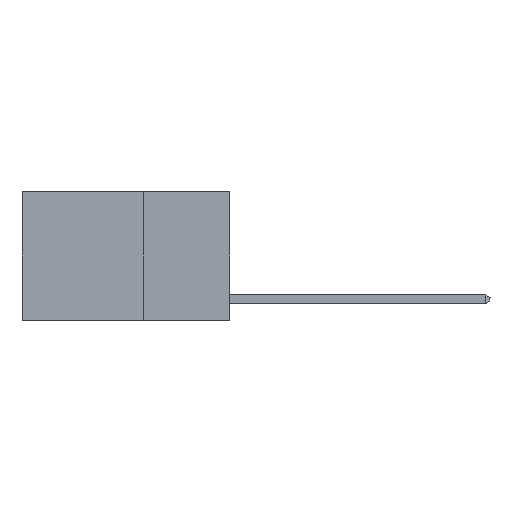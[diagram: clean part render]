
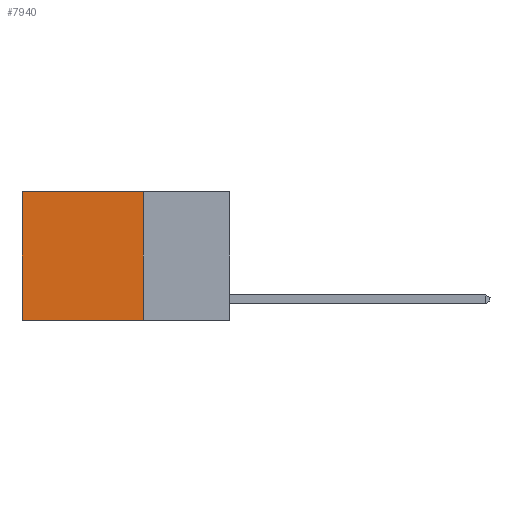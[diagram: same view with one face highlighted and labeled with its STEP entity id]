
A CAD part, left-side view. The second image highlights one B-rep face of the part: STEP entity #7940.
In plain terms, the highlighted planar face has unit normal (-1, 0, 0).
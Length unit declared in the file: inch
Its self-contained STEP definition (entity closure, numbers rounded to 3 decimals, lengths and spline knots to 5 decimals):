
#1257 = VECTOR ( 'NONE', #20396, 39.37008 ) ;
#1799 = CARTESIAN_POINT ( 'NONE',  ( 0.2625, 0.6, 0. ) ) ;
#1955 = VECTOR ( 'NONE', #23420, 39.37008 ) ;
#2367 = ORIENTED_EDGE ( 'NONE', *, *, #23529, .T. ) ;
#2864 = VECTOR ( 'NONE', #13400, 39.37008 ) ;
#3871 = VERTEX_POINT ( 'NONE', #1799 ) ;
#3995 = DIRECTION ( 'NONE',  ( 0., 0., -1. ) ) ;
#4753 = CARTESIAN_POINT ( 'NONE',  ( 0.2625, 0.25, 0. ) ) ;
#6244 = CARTESIAN_POINT ( 'NONE',  ( 0.2625, 0.25, 0. ) ) ;
#7244 = CARTESIAN_POINT ( 'NONE',  ( 0.2625, 0.6, -0.37 ) ) ;
#7940 = ADVANCED_FACE ( 'NONE', ( #25954 ), #25672, .F. ) ;
#8669 = LINE ( 'NONE', #17328, #1955 ) ;
#9231 = VERTEX_POINT ( 'NONE', #17182 ) ;
#9252 = EDGE_CURVE ( 'NONE', #9231, #19351, #8669, .T. ) ;
#9259 = VERTEX_POINT ( 'NONE', #19178 ) ;
#9519 = LINE ( 'NONE', #22286, #19576 ) ;
#10224 = DIRECTION ( 'NONE',  ( 1., 0., 0. ) ) ;
#13400 = DIRECTION ( 'NONE',  ( 0., 0., -1. ) ) ;
#14044 = LINE ( 'NONE', #26610, #1257 ) ;
#14243 = EDGE_CURVE ( 'NONE', #3871, #19351, #14044, .T. ) ;
#15891 = ORIENTED_EDGE ( 'NONE', *, *, #24357, .F. ) ;
#15917 = DIRECTION ( 'NONE',  ( 0., 1., 0. ) ) ;
#16016 = EDGE_LOOP ( 'NONE', ( #24887, #25338, #15891, #2367 ) ) ;
#17182 = CARTESIAN_POINT ( 'NONE',  ( 0.2625, 0.25, -0.37 ) ) ;
#17328 = CARTESIAN_POINT ( 'NONE',  ( 0.2625, 0.25, -0.37 ) ) ;
#19178 = CARTESIAN_POINT ( 'NONE',  ( 0.2625, 0.25, 0. ) ) ;
#19351 = VERTEX_POINT ( 'NONE', #7244 ) ;
#19576 = VECTOR ( 'NONE', #15917, 39.37008 ) ;
#19834 = AXIS2_PLACEMENT_3D ( 'NONE', #6244, #10224, #3995 ) ;
#20396 = DIRECTION ( 'NONE',  ( 0., 0., -1. ) ) ;
#22286 = CARTESIAN_POINT ( 'NONE',  ( 0.2625, 0.25, 0. ) ) ;
#23420 = DIRECTION ( 'NONE',  ( 0., 1., 0. ) ) ;
#23529 = EDGE_CURVE ( 'NONE', #9259, #3871, #9519, .T. ) ;
#24177 = LINE ( 'NONE', #4753, #2864 ) ;
#24357 = EDGE_CURVE ( 'NONE', #9259, #9231, #24177, .T. ) ;
#24887 = ORIENTED_EDGE ( 'NONE', *, *, #14243, .T. ) ;
#25338 = ORIENTED_EDGE ( 'NONE', *, *, #9252, .F. ) ;
#25672 = PLANE ( 'NONE',  #19834 ) ;
#25954 = FACE_OUTER_BOUND ( 'NONE', #16016, .T. ) ;
#26610 = CARTESIAN_POINT ( 'NONE',  ( 0.2625, 0.6, 0. ) ) ;
